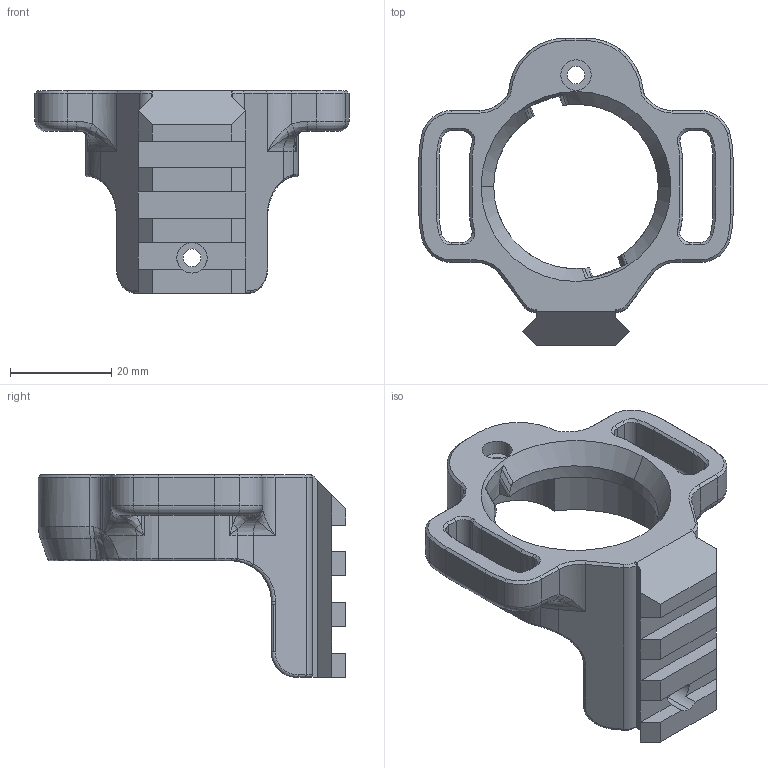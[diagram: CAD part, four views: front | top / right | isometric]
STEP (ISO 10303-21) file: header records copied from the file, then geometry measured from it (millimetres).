
FILE_DESCRIPTION (( 'STEP AP214' ), '1' );
FILE_NAME ('Sling_Point_V1.STEP', '2025-07-07T03:51:42', ( '' ), ( '' ), 'SwSTEP 2.0', 'SolidWorks 2020', '' );
FILE_SCHEMA (( 'AUTOMOTIVE_DESIGN' ));
Length unit declared in the file: millimetre
Products named in the file (1): Sling_Point_V1
Bounding box: 62 x 60.7 x 40 mm (x, y, z)
Volume: 18617.1 mm3; surface area: 10976.9 mm2
Topology: 1 solids, 1 shells, 323 faces, 793 edges, 464 vertices
Faces by surface type: cylinder 89, plane 88, bspline 71, cone 40, torus 35
Entity records: 12589 total; most frequent: CARTESIAN_POINT 5533, ORIENTED_EDGE 1572, DIRECTION 1337, EDGE_CURVE 786, AXIS2_PLACEMENT_3D 503, VERTEX_POINT 464, EDGE_LOOP 332, LINE 331
